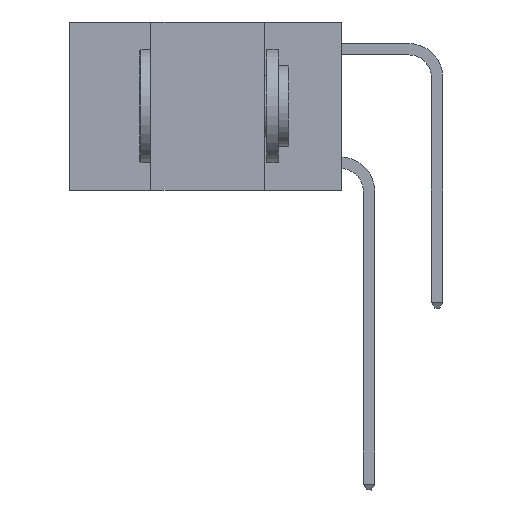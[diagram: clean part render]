
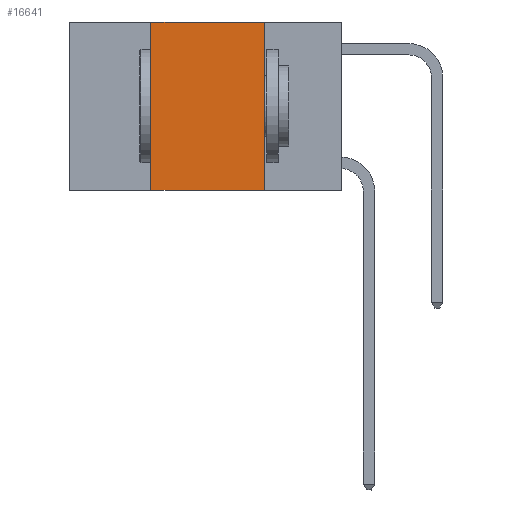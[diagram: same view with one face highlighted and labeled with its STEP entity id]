
A CAD part, left-side view. The second image highlights one B-rep face of the part: STEP entity #16641.
In plain terms, the highlighted planar face has unit normal (-1, 0, 0).
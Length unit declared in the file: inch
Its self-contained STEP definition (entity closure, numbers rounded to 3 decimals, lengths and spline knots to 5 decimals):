
#264 = EDGE_CURVE ( 'NONE', #7013, #26589, #3117, .T. ) ;
#707 = LINE ( 'NONE', #865, #17541 ) ;
#708 = DIRECTION ( 'NONE',  ( 0., 0., 1. ) ) ;
#865 = CARTESIAN_POINT ( 'NONE',  ( 0., 0.6, -0.37 ) ) ;
#892 = VERTEX_POINT ( 'NONE', #6866 ) ;
#1792 = CARTESIAN_POINT ( 'NONE',  ( 0., 0.17, -0.37 ) ) ;
#1793 = CARTESIAN_POINT ( 'NONE',  ( 0., 0.6, 0. ) ) ;
#2627 = LINE ( 'NONE', #21876, #8219 ) ;
#3117 = LINE ( 'NONE', #10836, #26257 ) ;
#3936 = DIRECTION ( 'NONE',  ( 1., 0., 0. ) ) ;
#4701 = FACE_OUTER_BOUND ( 'NONE', #25243, .T. ) ;
#5133 = ORIENTED_EDGE ( 'NONE', *, *, #12257, .F. ) ;
#6866 = CARTESIAN_POINT ( 'NONE',  ( 0., 0.17, 0. ) ) ;
#7013 = VERTEX_POINT ( 'NONE', #19877 ) ;
#7116 = DIRECTION ( 'NONE',  ( 0., 0., -1. ) ) ;
#7131 = DIRECTION ( 'NONE',  ( 0., -1., 0. ) ) ;
#8219 = VECTOR ( 'NONE', #7116, 39.37008 ) ;
#10213 = EDGE_CURVE ( 'NONE', #892, #13934, #2627, .T. ) ;
#10836 = CARTESIAN_POINT ( 'NONE',  ( 0., 0.42, 0. ) ) ;
#11391 = ORIENTED_EDGE ( 'NONE', *, *, #264, .F. ) ;
#12257 = EDGE_CURVE ( 'NONE', #26589, #892, #13383, .T. ) ;
#13383 = LINE ( 'NONE', #19762, #16455 ) ;
#13934 = VERTEX_POINT ( 'NONE', #1792 ) ;
#16236 = CARTESIAN_POINT ( 'NONE',  ( 0., 0.42, 0. ) ) ;
#16386 = EDGE_CURVE ( 'NONE', #7013, #13934, #707, .T. ) ;
#16455 = VECTOR ( 'NONE', #7131, 39.37008 ) ;
#16641 = ADVANCED_FACE ( 'NONE', ( #4701 ), #24983, .F. ) ;
#16986 = ORIENTED_EDGE ( 'NONE', *, *, #16386, .T. ) ;
#17541 = VECTOR ( 'NONE', #17755, 39.37008 ) ;
#17755 = DIRECTION ( 'NONE',  ( 0., -1., 0. ) ) ;
#18660 = DIRECTION ( 'NONE',  ( 0., 0., -1. ) ) ;
#19762 = CARTESIAN_POINT ( 'NONE',  ( 0., 0.6, 0. ) ) ;
#19877 = CARTESIAN_POINT ( 'NONE',  ( 0., 0.42, -0.37 ) ) ;
#20135 = AXIS2_PLACEMENT_3D ( 'NONE', #1793, #3936, #18660 ) ;
#21285 = ORIENTED_EDGE ( 'NONE', *, *, #10213, .F. ) ;
#21876 = CARTESIAN_POINT ( 'NONE',  ( 0., 0.17, 0. ) ) ;
#24983 = PLANE ( 'NONE',  #20135 ) ;
#25243 = EDGE_LOOP ( 'NONE', ( #21285, #5133, #11391, #16986 ) ) ;
#26257 = VECTOR ( 'NONE', #708, 39.37008 ) ;
#26589 = VERTEX_POINT ( 'NONE', #16236 ) ;
